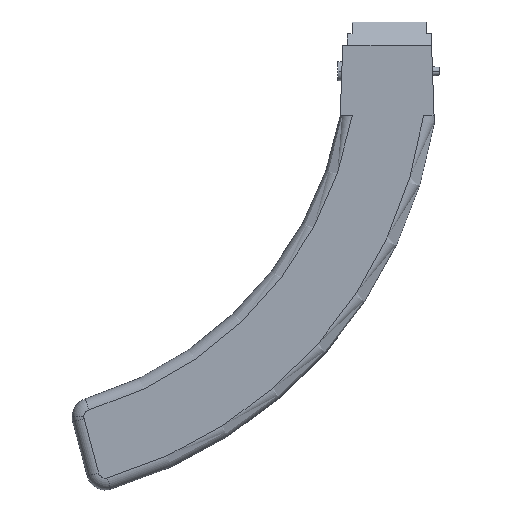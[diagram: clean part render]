
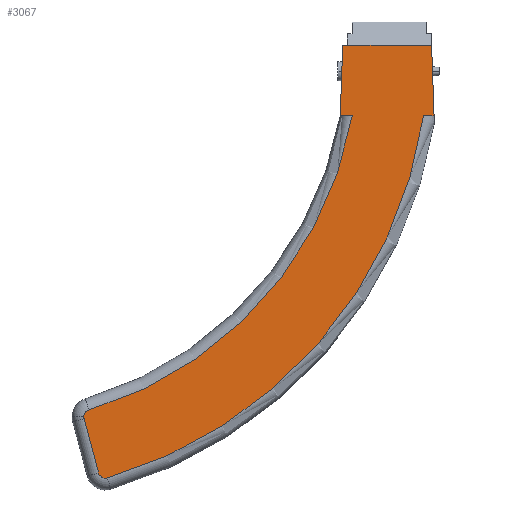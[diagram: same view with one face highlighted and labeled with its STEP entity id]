
A CAD part, top view. The second image highlights one B-rep face of the part: STEP entity #3067.
In plain terms, the highlighted planar face has unit normal (0, 0, 1).
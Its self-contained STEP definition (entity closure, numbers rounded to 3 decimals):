
#155 = DIRECTION ( 'NONE',  ( 1., 0., 0. ) ) ;
#183 = EDGE_CURVE ( 'NONE', #1173, #3645, #3726, .T. ) ;
#195 = DIRECTION ( 'NONE',  ( 1., 0., 0. ) ) ;
#243 = VERTEX_POINT ( 'NONE', #1441 ) ;
#513 = ORIENTED_EDGE ( 'NONE', *, *, #183, .F. ) ;
#547 = EDGE_CURVE ( 'NONE', #5172, #2814, #2998, .T. ) ;
#563 = VERTEX_POINT ( 'NONE', #4291 ) ;
#622 = AXIS2_PLACEMENT_3D ( 'NONE', #6286, #3245, #155 ) ;
#682 = DIRECTION ( 'NONE',  ( 0., 0., 1. ) ) ;
#751 = ORIENTED_EDGE ( 'NONE', *, *, #5809, .T. ) ;
#806 = CARTESIAN_POINT ( 'NONE',  ( -175., 0., 16. ) ) ;
#831 = CARTESIAN_POINT ( 'NONE',  ( -122.748, -179.552, 16. ) ) ;
#948 = ORIENTED_EDGE ( 'NONE', *, *, #1424, .T. ) ;
#1173 = VERTEX_POINT ( 'NONE', #2478 ) ;
#1300 = CARTESIAN_POINT ( 'NONE',  ( -131.859, -157.14, 16. ) ) ;
#1301 = DIRECTION ( 'NONE',  ( 1., 0., 0. ) ) ;
#1324 = DIRECTION ( 'NONE',  ( 1., 0., 0. ) ) ;
#1347 = DIRECTION ( 'NONE',  ( 1., 0., 0. ) ) ;
#1371 = LINE ( 'NONE', #3231, #2433 ) ;
#1424 = EDGE_CURVE ( 'NONE', #1598, #1758, #6621, .T. ) ;
#1441 = CARTESIAN_POINT ( 'NONE',  ( 12.926, -28., 16. ) ) ;
#1598 = VERTEX_POINT ( 'NONE', #1987 ) ;
#1643 = VECTOR ( 'NONE', #5964, 1000. ) ;
#1677 = EDGE_CURVE ( 'NONE', #563, #3120, #3671, .T. ) ;
#1680 = ORIENTED_EDGE ( 'NONE', *, *, #3209, .F. ) ;
#1758 = VERTEX_POINT ( 'NONE', #4499 ) ;
#1987 = CARTESIAN_POINT ( 'NONE',  ( -125.646, -180.328, 16. ) ) ;
#2179 = CIRCLE ( 'NONE', #5261, 190. ) ;
#2184 = AXIS2_PLACEMENT_3D ( 'NONE', #806, #4402, #1324 ) ;
#2314 = AXIS2_PLACEMENT_3D ( 'NONE', #831, #4421, #1347 ) ;
#2433 = VECTOR ( 'NONE', #2715, 1000. ) ;
#2440 = VERTEX_POINT ( 'NONE', #3690 ) ;
#2478 = CARTESIAN_POINT ( 'NONE',  ( -22.603, -28., 16. ) ) ;
#2495 = CARTESIAN_POINT ( 'NONE',  ( 16.349, 2., 16. ) ) ;
#2575 = ORIENTED_EDGE ( 'NONE', *, *, #547, .T. ) ;
#2605 = CIRCLE ( 'NONE', #622, 3. ) ;
#2608 = VECTOR ( 'NONE', #5730, 1000. ) ;
#2715 = DIRECTION ( 'NONE',  ( 0.259, -0.966, 0. ) ) ;
#2814 = VERTEX_POINT ( 'NONE', #2495 ) ;
#2827 = VECTOR ( 'NONE', #4766, 1000. ) ;
#2878 = CARTESIAN_POINT ( 'NONE',  ( -129.809, -153.485, 16. ) ) ;
#2997 = AXIS2_PLACEMENT_3D ( 'NONE', #3762, #682, #4271 ) ;
#2998 = LINE ( 'NONE', #5808, #2827 ) ;
#3067 = ADVANCED_FACE ( 'NONE', ( #3813 ), #5381, .T. ) ;
#3120 = VERTEX_POINT ( 'NONE', #2878 ) ;
#3172 = LINE ( 'NONE', #5450, #1643 ) ;
#3209 = EDGE_CURVE ( 'NONE', #5172, #243, #3172, .T. ) ;
#3219 = CARTESIAN_POINT ( 'NONE',  ( 17.397, -28., 16. ) ) ;
#3231 = CARTESIAN_POINT ( 'NONE',  ( -128.741, -168.778, 16. ) ) ;
#3245 = DIRECTION ( 'NONE',  ( 0., 0., 1. ) ) ;
#3270 = DIRECTION ( 'NONE',  ( 0., 0., 1. ) ) ;
#3355 = CARTESIAN_POINT ( 'NONE',  ( -129.707, -169.037, 16. ) ) ;
#3359 = CARTESIAN_POINT ( 'NONE',  ( 17.397, -28., 16. ) ) ;
#3394 = VECTOR ( 'NONE', #4611, 1000. ) ;
#3544 = EDGE_CURVE ( 'NONE', #2814, #3645, #3961, .T. ) ;
#3624 = EDGE_CURVE ( 'NONE', #2440, #4172, #5874, .T. ) ;
#3645 = VERTEX_POINT ( 'NONE', #5830 ) ;
#3671 = CIRCLE ( 'NONE', #2184, 160. ) ;
#3690 = CARTESIAN_POINT ( 'NONE',  ( -131.961, -156.363, 16. ) ) ;
#3726 = LINE ( 'NONE', #5100, #3394 ) ;
#3742 = DIRECTION ( 'NONE',  ( -1., 0., 0. ) ) ;
#3762 = CARTESIAN_POINT ( 'NONE',  ( -128.961, -156.363, 16. ) ) ;
#3813 = FACE_OUTER_BOUND ( 'NONE', #5943, .T. ) ;
#3961 = LINE ( 'NONE', #6207, #2608 ) ;
#4172 = VERTEX_POINT ( 'NONE', #1300 ) ;
#4271 = DIRECTION ( 'NONE',  ( 1., 0., 0. ) ) ;
#4289 = LINE ( 'NONE', #3219, #5149 ) ;
#4291 = CARTESIAN_POINT ( 'NONE',  ( -17.469, -28., 16. ) ) ;
#4381 = DIRECTION ( 'NONE',  ( 0., 0., 1. ) ) ;
#4402 = DIRECTION ( 'NONE',  ( 0., 0., -1. ) ) ;
#4421 = DIRECTION ( 'NONE',  ( 0., 0., 1. ) ) ;
#4469 = EDGE_CURVE ( 'NONE', #563, #1173, #4289, .T. ) ;
#4499 = CARTESIAN_POINT ( 'NONE',  ( -121.91, -182.432, 16. ) ) ;
#4611 = DIRECTION ( 'NONE',  ( 0.035, 0.999, 0. ) ) ;
#4766 = DIRECTION ( 'NONE',  ( -0.035, 0.999, 0. ) ) ;
#4852 = EDGE_CURVE ( 'NONE', #3120, #2440, #2605, .T. ) ;
#5094 = ORIENTED_EDGE ( 'NONE', *, *, #4852, .T. ) ;
#5100 = CARTESIAN_POINT ( 'NONE',  ( -21.508, 3.359, 16. ) ) ;
#5149 = VECTOR ( 'NONE', #3742, 1000. ) ;
#5172 = VERTEX_POINT ( 'NONE', #3359 ) ;
#5237 = AXIS2_PLACEMENT_3D ( 'NONE', #3355, #4381, #1301 ) ;
#5261 = AXIS2_PLACEMENT_3D ( 'NONE', #6321, #3270, #195 ) ;
#5381 = PLANE ( 'NONE',  #5237 ) ;
#5382 = ORIENTED_EDGE ( 'NONE', *, *, #4469, .F. ) ;
#5450 = CARTESIAN_POINT ( 'NONE',  ( 17.397, -28., 16. ) ) ;
#5467 = ORIENTED_EDGE ( 'NONE', *, *, #3544, .T. ) ;
#5625 = ORIENTED_EDGE ( 'NONE', *, *, #1677, .T. ) ;
#5730 = DIRECTION ( 'NONE',  ( -1., 0., 0. ) ) ;
#5808 = CARTESIAN_POINT ( 'NONE',  ( 16.35, 1.963, 16. ) ) ;
#5809 = EDGE_CURVE ( 'NONE', #4172, #1598, #1371, .T. ) ;
#5830 = CARTESIAN_POINT ( 'NONE',  ( -21.556, 2., 16. ) ) ;
#5874 = CIRCLE ( 'NONE', #2997, 3. ) ;
#5943 = EDGE_LOOP ( 'NONE', ( #6539, #1680, #2575, #5467, #513, #5382, #5625, #5094, #6083, #751, #948 ) ) ;
#5964 = DIRECTION ( 'NONE',  ( -1., 0., 0. ) ) ;
#6083 = ORIENTED_EDGE ( 'NONE', *, *, #3624, .T. ) ;
#6207 = CARTESIAN_POINT ( 'NONE',  ( 17.397, 2., 16. ) ) ;
#6286 = CARTESIAN_POINT ( 'NONE',  ( -128.961, -156.363, 16. ) ) ;
#6321 = CARTESIAN_POINT ( 'NONE',  ( -175., 0., 16. ) ) ;
#6539 = ORIENTED_EDGE ( 'NONE', *, *, #6615, .T. ) ;
#6615 = EDGE_CURVE ( 'NONE', #1758, #243, #2179, .T. ) ;
#6621 = CIRCLE ( 'NONE', #2314, 3. ) ;
